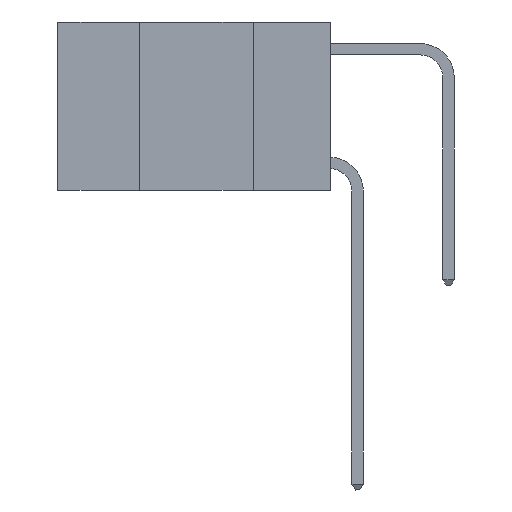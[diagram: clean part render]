
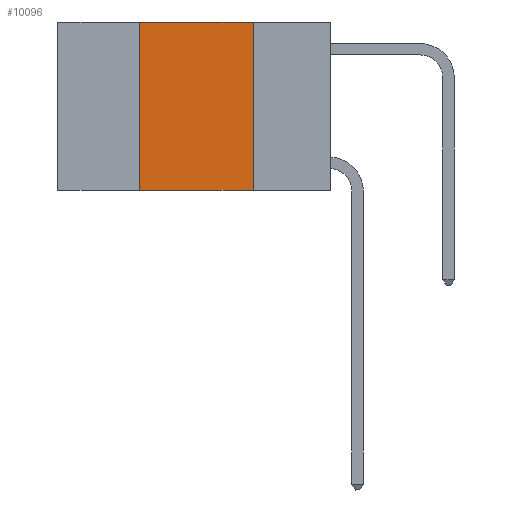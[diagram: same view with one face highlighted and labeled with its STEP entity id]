
A CAD part, left-side view. The second image highlights one B-rep face of the part: STEP entity #10096.
In plain terms, the highlighted planar face has unit normal (-1, 0, 0).
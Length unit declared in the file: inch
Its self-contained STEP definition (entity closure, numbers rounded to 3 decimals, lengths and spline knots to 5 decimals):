
#885 = LINE ( 'NONE', #16209, #5998 ) ;
#1685 = AXIS2_PLACEMENT_3D ( 'NONE', #3718, #9902, #15693 ) ;
#1693 = CARTESIAN_POINT ( 'NONE',  ( 0., 0.6, 0. ) ) ;
#1991 = CARTESIAN_POINT ( 'NONE',  ( 0., 0.6, -0.37 ) ) ;
#3311 = PLANE ( 'NONE',  #1685 ) ;
#3718 = CARTESIAN_POINT ( 'NONE',  ( 0., 0.6, 0. ) ) ;
#4154 = ORIENTED_EDGE ( 'NONE', *, *, #15956, .F. ) ;
#4848 = CARTESIAN_POINT ( 'NONE',  ( 0., 0.42, 0. ) ) ;
#5088 = ORIENTED_EDGE ( 'NONE', *, *, #15144, .T. ) ;
#5998 = VECTOR ( 'NONE', #17622, 39.37008 ) ;
#6175 = ORIENTED_EDGE ( 'NONE', *, *, #18651, .F. ) ;
#6595 = VERTEX_POINT ( 'NONE', #4848 ) ;
#7780 = DIRECTION ( 'NONE',  ( 0., -1., 0. ) ) ;
#8168 = DIRECTION ( 'NONE',  ( 0., -1., 0. ) ) ;
#8780 = VECTOR ( 'NONE', #8168, 39.37008 ) ;
#8988 = CARTESIAN_POINT ( 'NONE',  ( 0., 0.17, -0.37 ) ) ;
#9489 = CARTESIAN_POINT ( 'NONE',  ( 0., 0.42, -0.37 ) ) ;
#9620 = ORIENTED_EDGE ( 'NONE', *, *, #14955, .F. ) ;
#9902 = DIRECTION ( 'NONE',  ( 1., 0., 0. ) ) ;
#10096 = ADVANCED_FACE ( 'NONE', ( #19146 ), #3311, .F. ) ;
#11025 = LINE ( 'NONE', #1693, #14275 ) ;
#11061 = VECTOR ( 'NONE', #14294, 39.37008 ) ;
#12670 = LINE ( 'NONE', #16022, #11061 ) ;
#14275 = VECTOR ( 'NONE', #7780, 39.37008 ) ;
#14294 = DIRECTION ( 'NONE',  ( 0., 0., -1. ) ) ;
#14363 = CARTESIAN_POINT ( 'NONE',  ( 0., 0.17, 0. ) ) ;
#14944 = VERTEX_POINT ( 'NONE', #9489 ) ;
#14955 = EDGE_CURVE ( 'NONE', #6595, #18539, #11025, .T. ) ;
#15144 = EDGE_CURVE ( 'NONE', #14944, #18895, #19456, .T. ) ;
#15693 = DIRECTION ( 'NONE',  ( 0., 0., -1. ) ) ;
#15956 = EDGE_CURVE ( 'NONE', #18539, #18895, #12670, .T. ) ;
#16022 = CARTESIAN_POINT ( 'NONE',  ( 0., 0.17, 0. ) ) ;
#16209 = CARTESIAN_POINT ( 'NONE',  ( 0., 0.42, 0. ) ) ;
#17622 = DIRECTION ( 'NONE',  ( 0., 0., 1. ) ) ;
#17719 = EDGE_LOOP ( 'NONE', ( #4154, #9620, #6175, #5088 ) ) ;
#18539 = VERTEX_POINT ( 'NONE', #14363 ) ;
#18651 = EDGE_CURVE ( 'NONE', #14944, #6595, #885, .T. ) ;
#18895 = VERTEX_POINT ( 'NONE', #8988 ) ;
#19146 = FACE_OUTER_BOUND ( 'NONE', #17719, .T. ) ;
#19456 = LINE ( 'NONE', #1991, #8780 ) ;
